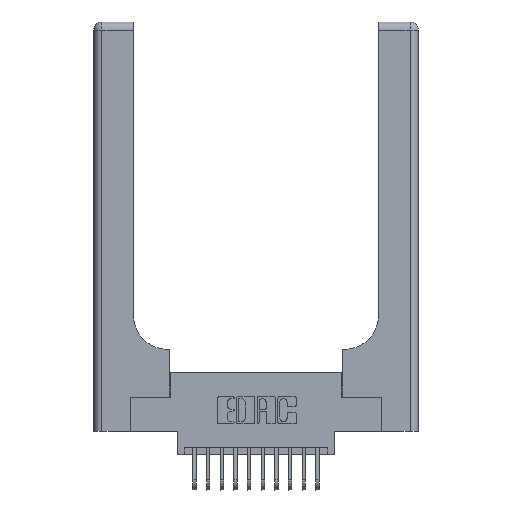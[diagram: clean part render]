
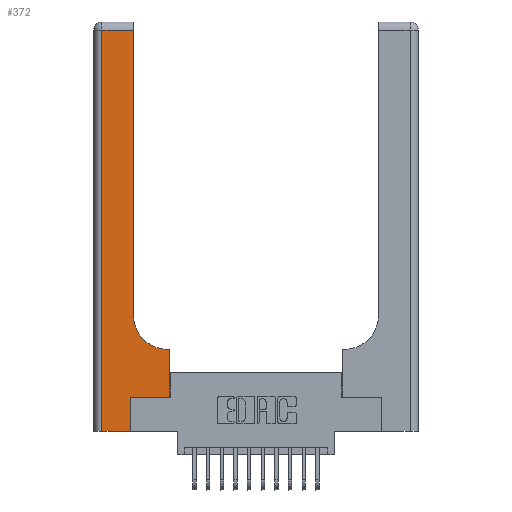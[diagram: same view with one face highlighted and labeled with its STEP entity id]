
A CAD part, top view. The second image highlights one B-rep face of the part: STEP entity #372.
In plain terms, the highlighted planar face has unit normal (0, 0, 1).
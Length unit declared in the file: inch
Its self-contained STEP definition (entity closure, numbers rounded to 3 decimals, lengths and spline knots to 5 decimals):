
#372 = ADVANCED_FACE ( 'NONE', ( #7811 ), #14336, .F. ) ;
#432 = EDGE_CURVE ( 'NONE', #11120, #14419, #6948, .T. ) ;
#1021 = DIRECTION ( 'NONE',  ( 1., 0., 0. ) ) ;
#1033 = CIRCLE ( 'NONE', #7573, 0.25 ) ;
#1297 = CARTESIAN_POINT ( 'NONE',  ( 0.06, 3., 0.37 ) ) ;
#1654 = VERTEX_POINT ( 'NONE', #5928 ) ;
#1717 = VECTOR ( 'NONE', #16836, 39.37008 ) ;
#2102 = ORIENTED_EDGE ( 'NONE', *, *, #5115, .T. ) ;
#2325 = DIRECTION ( 'NONE',  ( -1., 0., 0. ) ) ;
#2520 = DIRECTION ( 'NONE',  ( 0., 1., 0. ) ) ;
#2531 = LINE ( 'NONE', #3443, #13272 ) ;
#2719 = EDGE_CURVE ( 'NONE', #1654, #6640, #7580, .T. ) ;
#2989 = EDGE_LOOP ( 'NONE', ( #13418, #11567, #16022, #7206, #9770, #6365, #12035, #2102, #5107 ) ) ;
#3159 = EDGE_CURVE ( 'NONE', #6640, #4254, #4361, .T. ) ;
#3259 = EDGE_CURVE ( 'NONE', #4254, #11120, #6269, .T. ) ;
#3443 = CARTESIAN_POINT ( 'NONE',  ( 0.269, 0.25, 0.37 ) ) ;
#4064 = CARTESIAN_POINT ( 'NONE',  ( 0.2915, 3., 0.37 ) ) ;
#4131 = EDGE_CURVE ( 'NONE', #7424, #11833, #10678, .T. ) ;
#4254 = VERTEX_POINT ( 'NONE', #13559 ) ;
#4361 = LINE ( 'NONE', #16954, #4788 ) ;
#4788 = VECTOR ( 'NONE', #9184, 39.37008 ) ;
#5022 = CARTESIAN_POINT ( 'NONE',  ( 0., 0., 0.37 ) ) ;
#5107 = ORIENTED_EDGE ( 'NONE', *, *, #6247, .T. ) ;
#5115 = EDGE_CURVE ( 'NONE', #11833, #11004, #12071, .T. ) ;
#5818 = EDGE_CURVE ( 'NONE', #14419, #16988, #7893, .T. ) ;
#5907 = DIRECTION ( 'NONE',  ( 1., 0., 0. ) ) ;
#5928 = CARTESIAN_POINT ( 'NONE',  ( 0.2915, 0.85, 0.37 ) ) ;
#6247 = EDGE_CURVE ( 'NONE', #11004, #1654, #1033, .T. ) ;
#6269 = LINE ( 'NONE', #1297, #9469 ) ;
#6365 = ORIENTED_EDGE ( 'NONE', *, *, #6625, .T. ) ;
#6388 = CARTESIAN_POINT ( 'NONE',  ( 0., 3., 0.37 ) ) ;
#6625 = EDGE_CURVE ( 'NONE', #16988, #7424, #2531, .T. ) ;
#6640 = VERTEX_POINT ( 'NONE', #11600 ) ;
#6948 = LINE ( 'NONE', #5022, #13590 ) ;
#7206 = ORIENTED_EDGE ( 'NONE', *, *, #432, .T. ) ;
#7322 = CARTESIAN_POINT ( 'NONE',  ( 0.5585, 0.6, 0.37 ) ) ;
#7424 = VERTEX_POINT ( 'NONE', #15924 ) ;
#7471 = VECTOR ( 'NONE', #2520, 39.37008 ) ;
#7573 = AXIS2_PLACEMENT_3D ( 'NONE', #16976, #9201, #1021 ) ;
#7580 = LINE ( 'NONE', #4064, #14577 ) ;
#7811 = FACE_OUTER_BOUND ( 'NONE', #2989, .T. ) ;
#7893 = LINE ( 'NONE', #17109, #7471 ) ;
#8144 = DIRECTION ( 'NONE',  ( 0., 1., 0. ) ) ;
#9184 = DIRECTION ( 'NONE',  ( -1., 0., 0. ) ) ;
#9201 = DIRECTION ( 'NONE',  ( 0., 0., -1. ) ) ;
#9469 = VECTOR ( 'NONE', #10798, 39.37008 ) ;
#9770 = ORIENTED_EDGE ( 'NONE', *, *, #5818, .T. ) ;
#10471 = DIRECTION ( 'NONE',  ( 0., 0., -1. ) ) ;
#10678 = LINE ( 'NONE', #14554, #17150 ) ;
#10798 = DIRECTION ( 'NONE',  ( 0., -1., 0. ) ) ;
#11004 = VERTEX_POINT ( 'NONE', #15999 ) ;
#11120 = VERTEX_POINT ( 'NONE', #12346 ) ;
#11567 = ORIENTED_EDGE ( 'NONE', *, *, #3159, .T. ) ;
#11600 = CARTESIAN_POINT ( 'NONE',  ( 0.2915, 2.94, 0.37 ) ) ;
#11705 = CARTESIAN_POINT ( 'NONE',  ( 0.2915, 0.6, 0.37 ) ) ;
#11833 = VERTEX_POINT ( 'NONE', #7322 ) ;
#11894 = DIRECTION ( 'NONE',  ( 1., 0., 0. ) ) ;
#12035 = ORIENTED_EDGE ( 'NONE', *, *, #4131, .T. ) ;
#12071 = LINE ( 'NONE', #11705, #1717 ) ;
#12346 = CARTESIAN_POINT ( 'NONE',  ( 0.06, 0., 0.37 ) ) ;
#12480 = CARTESIAN_POINT ( 'NONE',  ( 0.269, 0.25, 0.37 ) ) ;
#13272 = VECTOR ( 'NONE', #5907, 39.37008 ) ;
#13418 = ORIENTED_EDGE ( 'NONE', *, *, #2719, .T. ) ;
#13559 = CARTESIAN_POINT ( 'NONE',  ( 0.06, 2.94, 0.37 ) ) ;
#13590 = VECTOR ( 'NONE', #11894, 39.37008 ) ;
#14229 = CARTESIAN_POINT ( 'NONE',  ( 0.269, 0., 0.37 ) ) ;
#14336 = PLANE ( 'NONE',  #15159 ) ;
#14419 = VERTEX_POINT ( 'NONE', #14229 ) ;
#14554 = CARTESIAN_POINT ( 'NONE',  ( 0.5585, 0.25, 0.37 ) ) ;
#14577 = VECTOR ( 'NONE', #8144, 39.37008 ) ;
#15159 = AXIS2_PLACEMENT_3D ( 'NONE', #6388, #10471, #2325 ) ;
#15838 = DIRECTION ( 'NONE',  ( 0., 1., 0. ) ) ;
#15924 = CARTESIAN_POINT ( 'NONE',  ( 0.5585, 0.25, 0.37 ) ) ;
#15999 = CARTESIAN_POINT ( 'NONE',  ( 0.5415, 0.6, 0.37 ) ) ;
#16022 = ORIENTED_EDGE ( 'NONE', *, *, #3259, .T. ) ;
#16836 = DIRECTION ( 'NONE',  ( -1., 0., 0. ) ) ;
#16954 = CARTESIAN_POINT ( 'NONE',  ( 0., 2.94, 0.37 ) ) ;
#16976 = CARTESIAN_POINT ( 'NONE',  ( 0.5415, 0.85, 0.37 ) ) ;
#16988 = VERTEX_POINT ( 'NONE', #12480 ) ;
#17109 = CARTESIAN_POINT ( 'NONE',  ( 0.269, 0., 0.37 ) ) ;
#17150 = VECTOR ( 'NONE', #15838, 39.37008 ) ;
